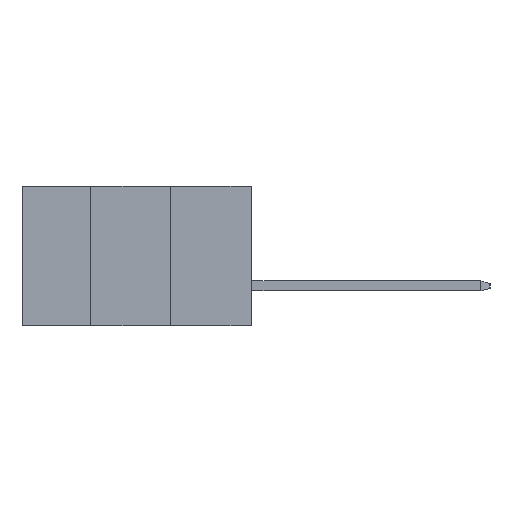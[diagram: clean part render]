
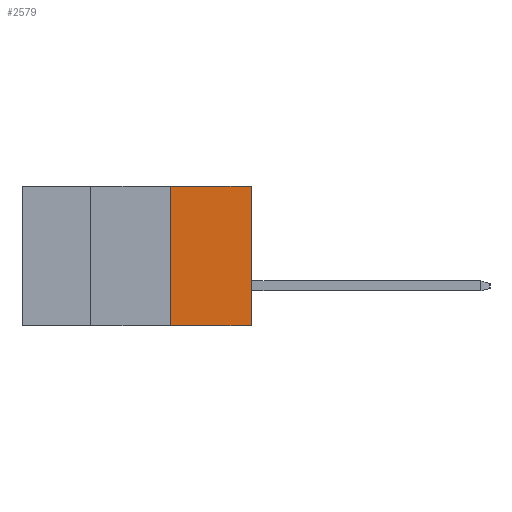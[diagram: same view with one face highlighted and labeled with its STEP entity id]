
A CAD part, left-side view. The second image highlights one B-rep face of the part: STEP entity #2579.
In plain terms, the highlighted planar face has unit normal (-1, 0, 0).
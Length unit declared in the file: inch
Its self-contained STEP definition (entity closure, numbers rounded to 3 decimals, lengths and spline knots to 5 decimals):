
#150 = DIRECTION ( 'NONE',  ( 1., 0., 0. ) ) ;
#166 = CARTESIAN_POINT ( 'NONE',  ( 0.4265, 0.254, -0.437 ) ) ;
#417 = LINE ( 'NONE', #7261, #7392 ) ;
#596 = EDGE_CURVE ( 'NONE', #2151, #11907, #417, .T. ) ;
#893 = LINE ( 'NONE', #1793, #2606 ) ;
#969 = CARTESIAN_POINT ( 'NONE',  ( 0.4265, 0., -0.437 ) ) ;
#1181 = EDGE_LOOP ( 'NONE', ( #5023, #11761, #2075, #5885 ) ) ;
#1793 = CARTESIAN_POINT ( 'NONE',  ( 0.4265, 0.254, 0. ) ) ;
#1847 = EDGE_CURVE ( 'NONE', #2151, #4321, #10272, .T. ) ;
#2075 = ORIENTED_EDGE ( 'NONE', *, *, #596, .F. ) ;
#2151 = VERTEX_POINT ( 'NONE', #166 ) ;
#2293 = CARTESIAN_POINT ( 'NONE',  ( 0.4265, 0.254, -0.437 ) ) ;
#2579 = ADVANCED_FACE ( 'NONE', ( #5016 ), #11866, .F. ) ;
#2606 = VECTOR ( 'NONE', #4608, 39.37008 ) ;
#2926 = VECTOR ( 'NONE', #6437, 39.37008 ) ;
#4133 = CARTESIAN_POINT ( 'NONE',  ( 0.4265, 0.254, 0. ) ) ;
#4321 = VERTEX_POINT ( 'NONE', #5507 ) ;
#4608 = DIRECTION ( 'NONE',  ( 0., -1., 0. ) ) ;
#5016 = FACE_OUTER_BOUND ( 'NONE', #1181, .T. ) ;
#5023 = ORIENTED_EDGE ( 'NONE', *, *, #7386, .T. ) ;
#5507 = CARTESIAN_POINT ( 'NONE',  ( 0.4265, 0., -0.437 ) ) ;
#5885 = ORIENTED_EDGE ( 'NONE', *, *, #1847, .T. ) ;
#5944 = DIRECTION ( 'NONE',  ( 0., 0., 1. ) ) ;
#6050 = EDGE_CURVE ( 'NONE', #11907, #9223, #893, .T. ) ;
#6437 = DIRECTION ( 'NONE',  ( 0., -1., 0. ) ) ;
#7261 = CARTESIAN_POINT ( 'NONE',  ( 0.4265, 0.254, -0.437 ) ) ;
#7386 = EDGE_CURVE ( 'NONE', #4321, #9223, #11966, .T. ) ;
#7392 = VECTOR ( 'NONE', #11236, 39.37008 ) ;
#7715 = CARTESIAN_POINT ( 'NONE',  ( 0.4265, 0., 0. ) ) ;
#7953 = DIRECTION ( 'NONE',  ( 0., 0., -1. ) ) ;
#8914 = CARTESIAN_POINT ( 'NONE',  ( 0.4265, 0.254, -0.437 ) ) ;
#9223 = VERTEX_POINT ( 'NONE', #7715 ) ;
#10272 = LINE ( 'NONE', #2293, #2926 ) ;
#11236 = DIRECTION ( 'NONE',  ( 0., 0., 1. ) ) ;
#11402 = VECTOR ( 'NONE', #5944, 39.37008 ) ;
#11761 = ORIENTED_EDGE ( 'NONE', *, *, #6050, .F. ) ;
#11866 = PLANE ( 'NONE',  #11967 ) ;
#11907 = VERTEX_POINT ( 'NONE', #4133 ) ;
#11966 = LINE ( 'NONE', #969, #11402 ) ;
#11967 = AXIS2_PLACEMENT_3D ( 'NONE', #8914, #150, #7953 ) ;
